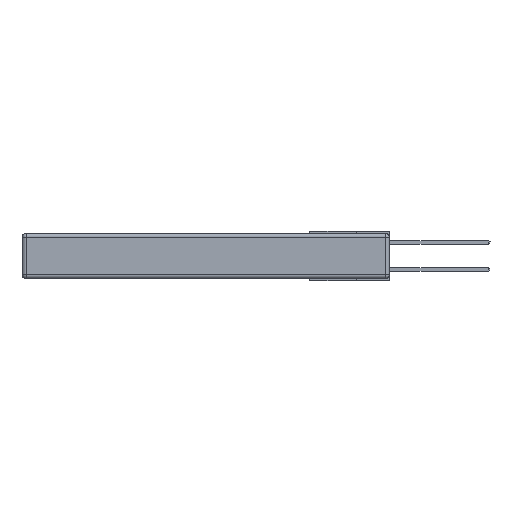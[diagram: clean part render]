
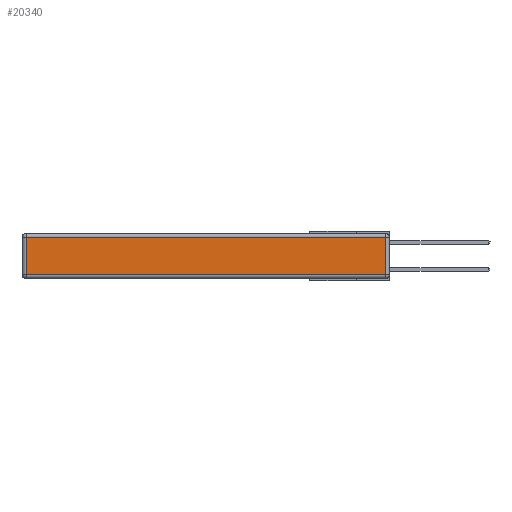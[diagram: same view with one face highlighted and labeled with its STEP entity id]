
A CAD part, left-side view. The second image highlights one B-rep face of the part: STEP entity #20340.
In plain terms, the highlighted planar face has unit normal (-1, 0, 0).
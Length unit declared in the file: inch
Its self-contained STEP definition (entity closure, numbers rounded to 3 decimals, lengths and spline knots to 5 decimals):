
#215 = CARTESIAN_POINT ( 'NONE',  ( 0., 0., -0.313 ) ) ;
#230 = CARTESIAN_POINT ( 'NONE',  ( 0., 0.03, -0.343 ) ) ;
#1736 = DIRECTION ( 'NONE',  ( 0., 0., -1. ) ) ;
#2056 = EDGE_CURVE ( 'NONE', #20813, #10097, #22086, .T. ) ;
#2558 = DIRECTION ( 'NONE',  ( -1., 0., 0. ) ) ;
#2907 = EDGE_CURVE ( 'NONE', #9830, #10608, #20464, .T. ) ;
#3305 = LINE ( 'NONE', #215, #6836 ) ;
#5349 = EDGE_LOOP ( 'NONE', ( #19099, #7220, #13875, #20753 ) ) ;
#6146 = DIRECTION ( 'NONE',  ( 0., 0., 1. ) ) ;
#6836 = VECTOR ( 'NONE', #16513, 39.37008 ) ;
#6988 = DIRECTION ( 'NONE',  ( 0., 1., 0. ) ) ;
#7220 = ORIENTED_EDGE ( 'NONE', *, *, #2907, .T. ) ;
#7333 = CARTESIAN_POINT ( 'NONE',  ( 0., 2.75, -0.03 ) ) ;
#8797 = FACE_OUTER_BOUND ( 'NONE', #5349, .T. ) ;
#9830 = VERTEX_POINT ( 'NONE', #16973 ) ;
#10097 = VERTEX_POINT ( 'NONE', #24192 ) ;
#10608 = VERTEX_POINT ( 'NONE', #24676 ) ;
#11914 = AXIS2_PLACEMENT_3D ( 'NONE', #14752, #2558, #14928 ) ;
#13115 = CARTESIAN_POINT ( 'NONE',  ( 0., 2.72, -0.03 ) ) ;
#13875 = ORIENTED_EDGE ( 'NONE', *, *, #14202, .T. ) ;
#14202 = EDGE_CURVE ( 'NONE', #10608, #20813, #23205, .T. ) ;
#14666 = PLANE ( 'NONE',  #11914 ) ;
#14752 = CARTESIAN_POINT ( 'NONE',  ( 0., 0., -0.343 ) ) ;
#14928 = DIRECTION ( 'NONE',  ( 0., 0., 1. ) ) ;
#16513 = DIRECTION ( 'NONE',  ( 0., -1., 0. ) ) ;
#16973 = CARTESIAN_POINT ( 'NONE',  ( 0., 0.03, -0.313 ) ) ;
#18309 = CARTESIAN_POINT ( 'NONE',  ( 0., 2.72, -0.343 ) ) ;
#18891 = VECTOR ( 'NONE', #6146, 39.37008 ) ;
#19099 = ORIENTED_EDGE ( 'NONE', *, *, #21265, .T. ) ;
#20340 = ADVANCED_FACE ( 'NONE', ( #8797 ), #14666, .T. ) ;
#20464 = LINE ( 'NONE', #230, #18891 ) ;
#20753 = ORIENTED_EDGE ( 'NONE', *, *, #2056, .T. ) ;
#20813 = VERTEX_POINT ( 'NONE', #13115 ) ;
#21265 = EDGE_CURVE ( 'NONE', #10097, #9830, #3305, .T. ) ;
#22086 = LINE ( 'NONE', #18309, #23977 ) ;
#23205 = LINE ( 'NONE', #7333, #25120 ) ;
#23977 = VECTOR ( 'NONE', #1736, 39.37008 ) ;
#24192 = CARTESIAN_POINT ( 'NONE',  ( 0., 2.72, -0.313 ) ) ;
#24676 = CARTESIAN_POINT ( 'NONE',  ( 0., 0.03, -0.03 ) ) ;
#25120 = VECTOR ( 'NONE', #6988, 39.37008 ) ;
